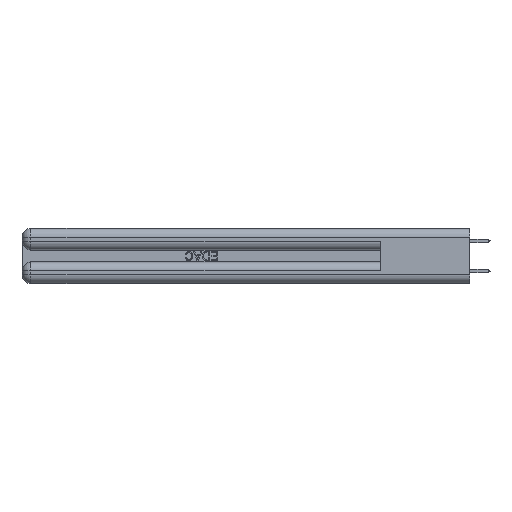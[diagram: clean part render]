
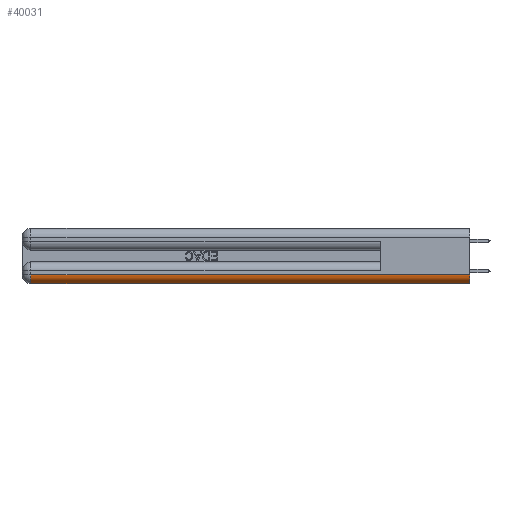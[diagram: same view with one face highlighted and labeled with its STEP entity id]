
A CAD part, left-side view. The second image highlights one B-rep face of the part: STEP entity #40031.
In plain terms, the highlighted cylindrical face has radius 1.524 mm (diameter 3.048 mm), a partial arc.
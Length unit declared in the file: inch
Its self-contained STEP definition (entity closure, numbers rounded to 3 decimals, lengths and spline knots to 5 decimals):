
#2550 = CARTESIAN_POINT ( 'NONE',  ( 0.06, 2.94, 0.06 ) ) ;
#5213 = DIRECTION ( 'NONE',  ( 0., 1., 0. ) ) ;
#5294 = CARTESIAN_POINT ( 'NONE',  ( 0.06, 0., 0.06 ) ) ;
#6223 = DIRECTION ( 'NONE',  ( 0., 0., 1. ) ) ;
#8384 = VERTEX_POINT ( 'NONE', #47162 ) ;
#8639 = AXIS2_PLACEMENT_3D ( 'NONE', #2550, #28059, #6223 ) ;
#8984 = DIRECTION ( 'NONE',  ( 0., 0., 1. ) ) ;
#13030 = VECTOR ( 'NONE', #5213, 39.37008 ) ;
#15577 = VECTOR ( 'NONE', #41561, 39.37008 ) ;
#16660 = FACE_OUTER_BOUND ( 'NONE', #32961, .T. ) ;
#17070 = CARTESIAN_POINT ( 'NONE',  ( 0.06, 0., 0.06 ) ) ;
#17611 = CARTESIAN_POINT ( 'NONE',  ( 0., 2.94, 0.06 ) ) ;
#19638 = EDGE_CURVE ( 'NONE', #8384, #29551, #21083, .T. ) ;
#20727 = DIRECTION ( 'NONE',  ( 0., 0., 1. ) ) ;
#21083 = CIRCLE ( 'NONE', #25335, 0.06 ) ;
#21546 = LINE ( 'NONE', #27058, #13030 ) ;
#23258 = VERTEX_POINT ( 'NONE', #44532 ) ;
#25335 = AXIS2_PLACEMENT_3D ( 'NONE', #5294, #30802, #8984 ) ;
#26185 = VERTEX_POINT ( 'NONE', #17611 ) ;
#26502 = ORIENTED_EDGE ( 'NONE', *, *, #19638, .F. ) ;
#27058 = CARTESIAN_POINT ( 'NONE',  ( 0.06, 3., 0. ) ) ;
#28059 = DIRECTION ( 'NONE',  ( 0., 1., 0. ) ) ;
#29551 = VERTEX_POINT ( 'NONE', #33403 ) ;
#30740 = ORIENTED_EDGE ( 'NONE', *, *, #37953, .F. ) ;
#30749 = CARTESIAN_POINT ( 'NONE',  ( 0., 0., 0.06 ) ) ;
#30802 = DIRECTION ( 'NONE',  ( 0., -1., 0. ) ) ;
#32405 = ORIENTED_EDGE ( 'NONE', *, *, #34736, .F. ) ;
#32961 = EDGE_LOOP ( 'NONE', ( #26502, #32405, #30740, #42398 ) ) ;
#33403 = CARTESIAN_POINT ( 'NONE',  ( 0.06, 0., 0. ) ) ;
#34736 = EDGE_CURVE ( 'NONE', #26185, #8384, #43489, .T. ) ;
#34863 = CYLINDRICAL_SURFACE ( 'NONE', #43171, 0.06 ) ;
#37953 = EDGE_CURVE ( 'NONE', #23258, #26185, #44303, .T. ) ;
#38874 = DIRECTION ( 'NONE',  ( 0., 1., 0. ) ) ;
#40031 = ADVANCED_FACE ( 'NONE', ( #16660 ), #34863, .T. ) ;
#41561 = DIRECTION ( 'NONE',  ( 0., -1., 0. ) ) ;
#42398 = ORIENTED_EDGE ( 'NONE', *, *, #42449, .F. ) ;
#42449 = EDGE_CURVE ( 'NONE', #29551, #23258, #21546, .T. ) ;
#43171 = AXIS2_PLACEMENT_3D ( 'NONE', #17070, #38874, #20727 ) ;
#43489 = LINE ( 'NONE', #30749, #15577 ) ;
#44303 = CIRCLE ( 'NONE', #8639, 0.06 ) ;
#44532 = CARTESIAN_POINT ( 'NONE',  ( 0.06, 2.94, 0. ) ) ;
#47162 = CARTESIAN_POINT ( 'NONE',  ( 0., 0., 0.06 ) ) ;
